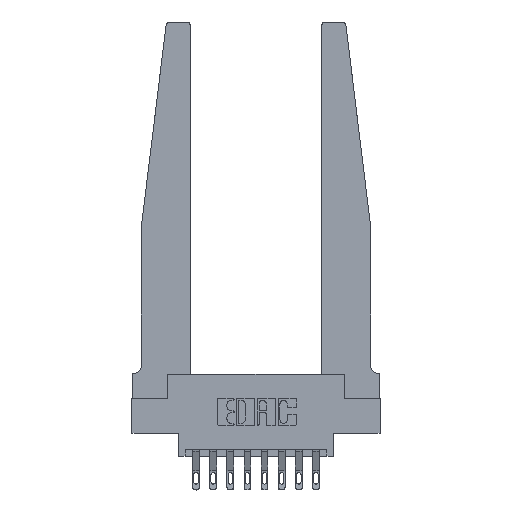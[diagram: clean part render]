
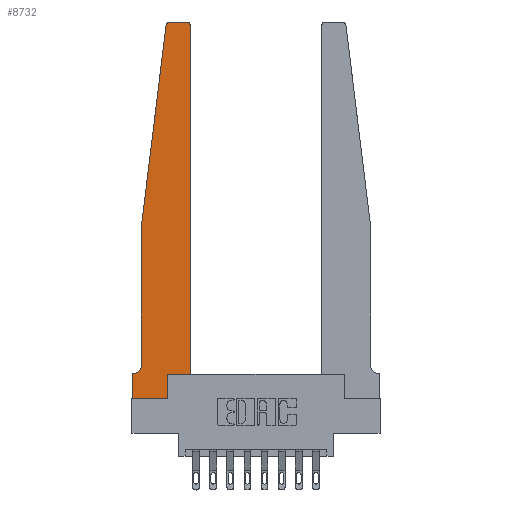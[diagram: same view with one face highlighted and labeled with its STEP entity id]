
A CAD part, top view. The second image highlights one B-rep face of the part: STEP entity #8732.
In plain terms, the highlighted planar face has unit normal (0, 0, 1).
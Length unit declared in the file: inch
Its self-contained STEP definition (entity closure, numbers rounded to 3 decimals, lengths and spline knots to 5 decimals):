
#135 = ORIENTED_EDGE ( 'NONE', *, *, #14072, .T. ) ;
#791 = ORIENTED_EDGE ( 'NONE', *, *, #9871, .T. ) ;
#816 = VERTEX_POINT ( 'NONE', #8005 ) ;
#906 = CARTESIAN_POINT ( 'NONE',  ( 0., 0., 0.37 ) ) ;
#1150 = ORIENTED_EDGE ( 'NONE', *, *, #10931, .T. ) ;
#1225 = CIRCLE ( 'NONE', #9294, 0.03 ) ;
#1299 = LINE ( 'NONE', #4292, #7517 ) ;
#1428 = VECTOR ( 'NONE', #4726, 39.37008 ) ;
#1521 = CARTESIAN_POINT ( 'NONE',  ( 0.015, 0.1875, 0.37 ) ) ;
#1826 = AXIS2_PLACEMENT_3D ( 'NONE', #9132, #2175, #10314 ) ;
#1979 = DIRECTION ( 'NONE',  ( 0., 1., 0. ) ) ;
#2053 = CARTESIAN_POINT ( 'NONE',  ( 0.2605, 0., 0.37 ) ) ;
#2154 = VERTEX_POINT ( 'NONE', #10411 ) ;
#2175 = DIRECTION ( 'NONE',  ( 0., 0., 1. ) ) ;
#2312 = EDGE_CURVE ( 'NONE', #8022, #6058, #6908, .T. ) ;
#2377 = AXIS2_PLACEMENT_3D ( 'NONE', #6183, #2747, #10862 ) ;
#2577 = VERTEX_POINT ( 'NONE', #13410 ) ;
#2712 = CARTESIAN_POINT ( 'NONE',  ( 0.395, 2.75, 0.37 ) ) ;
#2747 = DIRECTION ( 'NONE',  ( 0., 0., 1. ) ) ;
#2758 = EDGE_CURVE ( 'NONE', #9063, #12948, #14147, .T. ) ;
#2855 = DIRECTION ( 'NONE',  ( -1., 0., 0. ) ) ;
#3118 = FACE_OUTER_BOUND ( 'NONE', #8728, .T. ) ;
#3234 = VECTOR ( 'NONE', #10538, 39.37008 ) ;
#3878 = VERTEX_POINT ( 'NONE', #11262 ) ;
#3969 = LINE ( 'NONE', #9019, #9789 ) ;
#3989 = EDGE_CURVE ( 'NONE', #6770, #14047, #14285, .T. ) ;
#4067 = AXIS2_PLACEMENT_3D ( 'NONE', #11830, #4879, #12987 ) ;
#4113 = ORIENTED_EDGE ( 'NONE', *, *, #11872, .T. ) ;
#4292 = CARTESIAN_POINT ( 'NONE',  ( 0.425, 0.18, 0.37 ) ) ;
#4310 = VECTOR ( 'NONE', #10829, 39.37008 ) ;
#4442 = LINE ( 'NONE', #9015, #10245 ) ;
#4726 = DIRECTION ( 'NONE',  ( 0., 1., 0. ) ) ;
#4879 = DIRECTION ( 'NONE',  ( 0., 0., -1. ) ) ;
#5049 = CARTESIAN_POINT ( 'NONE',  ( 0.065, 0.1875, 0.37 ) ) ;
#6058 = VERTEX_POINT ( 'NONE', #1521 ) ;
#6165 = VERTEX_POINT ( 'NONE', #8687 ) ;
#6183 = CARTESIAN_POINT ( 'NONE',  ( 0., 0.1875, 0.37 ) ) ;
#6198 = DIRECTION ( 'NONE',  ( 0., 0., 1. ) ) ;
#6335 = CARTESIAN_POINT ( 'NONE',  ( 0.2605, 0.18, 0.37 ) ) ;
#6716 = CARTESIAN_POINT ( 'NONE',  ( 0.425, 0.18, 0.37 ) ) ;
#6770 = VERTEX_POINT ( 'NONE', #14571 ) ;
#6908 = CIRCLE ( 'NONE', #4067, 0.05 ) ;
#6927 = EDGE_CURVE ( 'NONE', #816, #2154, #4442, .T. ) ;
#7020 = LINE ( 'NONE', #5049, #4310 ) ;
#7452 = EDGE_CURVE ( 'NONE', #12948, #10069, #1299, .T. ) ;
#7517 = VECTOR ( 'NONE', #11233, 39.37008 ) ;
#7674 = VECTOR ( 'NONE', #2855, 39.37008 ) ;
#7788 = CARTESIAN_POINT ( 'NONE',  ( 0.425, 0.18, 0.37 ) ) ;
#7846 = VECTOR ( 'NONE', #1979, 39.37008 ) ;
#8005 = CARTESIAN_POINT ( 'NONE',  ( 0.24675, 2.72367, 0.37 ) ) ;
#8022 = VERTEX_POINT ( 'NONE', #14691 ) ;
#8119 = ORIENTED_EDGE ( 'NONE', *, *, #8400, .T. ) ;
#8183 = EDGE_CURVE ( 'NONE', #14047, #3878, #10401, .T. ) ;
#8400 = EDGE_CURVE ( 'NONE', #10069, #6770, #12032, .T. ) ;
#8687 = CARTESIAN_POINT ( 'NONE',  ( 0., 0., 0.37 ) ) ;
#8728 = EDGE_LOOP ( 'NONE', ( #12248, #791, #11130, #1150, #13368, #135, #4113, #12514, #13993, #13391, #8119, #9500 ) ) ;
#8732 = ADVANCED_FACE ( 'NONE', ( #3118 ), #9704, .T. ) ;
#9015 = CARTESIAN_POINT ( 'NONE',  ( 0.065, 1.25, 0.37 ) ) ;
#9019 = CARTESIAN_POINT ( 'NONE',  ( 0., 0., 0.37 ) ) ;
#9032 = VECTOR ( 'NONE', #12574, 39.37008 ) ;
#9063 = VERTEX_POINT ( 'NONE', #2053 ) ;
#9132 = CARTESIAN_POINT ( 'NONE',  ( 0.395, 2.72, 0.37 ) ) ;
#9294 = AXIS2_PLACEMENT_3D ( 'NONE', #13149, #6198, #14297 ) ;
#9317 = CARTESIAN_POINT ( 'NONE',  ( 0.2605, 0.18, 0.37 ) ) ;
#9500 = ORIENTED_EDGE ( 'NONE', *, *, #3989, .T. ) ;
#9704 = PLANE ( 'NONE',  #2377 ) ;
#9789 = VECTOR ( 'NONE', #10198, 39.37008 ) ;
#9820 = CARTESIAN_POINT ( 'NONE',  ( 0.25, 2.75, 0.37 ) ) ;
#9871 = EDGE_CURVE ( 'NONE', #3878, #816, #1225, .T. ) ;
#10069 = VERTEX_POINT ( 'NONE', #6716 ) ;
#10198 = DIRECTION ( 'NONE',  ( 1., 0., 0. ) ) ;
#10245 = VECTOR ( 'NONE', #12580, 39.37008 ) ;
#10314 = DIRECTION ( 'NONE',  ( 1., 0., 0. ) ) ;
#10401 = LINE ( 'NONE', #9820, #7674 ) ;
#10411 = CARTESIAN_POINT ( 'NONE',  ( 0.065, 1.25, 0.37 ) ) ;
#10538 = DIRECTION ( 'NONE',  ( 0., -1., 0. ) ) ;
#10829 = DIRECTION ( 'NONE',  ( -1., 0., 0. ) ) ;
#10862 = DIRECTION ( 'NONE',  ( 1., 0., 0. ) ) ;
#10931 = EDGE_CURVE ( 'NONE', #2154, #8022, #12133, .T. ) ;
#11130 = ORIENTED_EDGE ( 'NONE', *, *, #6927, .T. ) ;
#11233 = DIRECTION ( 'NONE',  ( 1., 0., 0. ) ) ;
#11262 = CARTESIAN_POINT ( 'NONE',  ( 0.27653, 2.75, 0.37 ) ) ;
#11751 = CARTESIAN_POINT ( 'NONE',  ( 0.065, 1.25, 0.37 ) ) ;
#11830 = CARTESIAN_POINT ( 'NONE',  ( 0.015, 0.2375, 0.37 ) ) ;
#11872 = EDGE_CURVE ( 'NONE', #2577, #6165, #13739, .T. ) ;
#12032 = LINE ( 'NONE', #7788, #7846 ) ;
#12133 = LINE ( 'NONE', #11751, #3234 ) ;
#12248 = ORIENTED_EDGE ( 'NONE', *, *, #8183, .T. ) ;
#12514 = ORIENTED_EDGE ( 'NONE', *, *, #13124, .T. ) ;
#12574 = DIRECTION ( 'NONE',  ( 0., -1., 0. ) ) ;
#12580 = DIRECTION ( 'NONE',  ( -0.122, -0.992, 0. ) ) ;
#12948 = VERTEX_POINT ( 'NONE', #6335 ) ;
#12987 = DIRECTION ( 'NONE',  ( -1., 0., 0. ) ) ;
#13124 = EDGE_CURVE ( 'NONE', #6165, #9063, #3969, .T. ) ;
#13149 = CARTESIAN_POINT ( 'NONE',  ( 0.27653, 2.72, 0.37 ) ) ;
#13368 = ORIENTED_EDGE ( 'NONE', *, *, #2312, .T. ) ;
#13391 = ORIENTED_EDGE ( 'NONE', *, *, #7452, .T. ) ;
#13410 = CARTESIAN_POINT ( 'NONE',  ( 0., 0.1875, 0.37 ) ) ;
#13739 = LINE ( 'NONE', #906, #9032 ) ;
#13993 = ORIENTED_EDGE ( 'NONE', *, *, #2758, .T. ) ;
#14047 = VERTEX_POINT ( 'NONE', #2712 ) ;
#14072 = EDGE_CURVE ( 'NONE', #6058, #2577, #7020, .T. ) ;
#14147 = LINE ( 'NONE', #9317, #1428 ) ;
#14285 = CIRCLE ( 'NONE', #1826, 0.03 ) ;
#14297 = DIRECTION ( 'NONE',  ( 1., 0., 0. ) ) ;
#14571 = CARTESIAN_POINT ( 'NONE',  ( 0.425, 2.72, 0.37 ) ) ;
#14691 = CARTESIAN_POINT ( 'NONE',  ( 0.065, 0.2375, 0.37 ) ) ;
